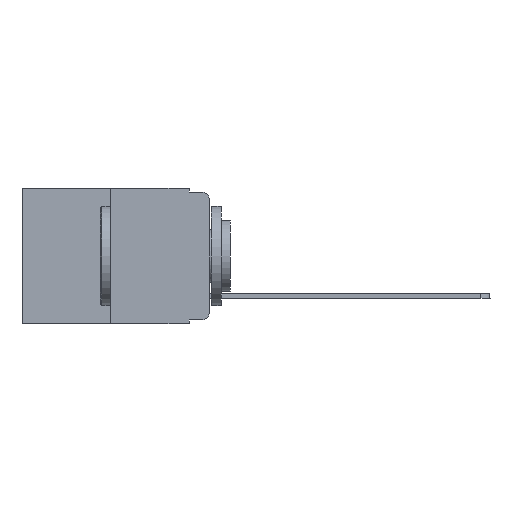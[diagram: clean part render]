
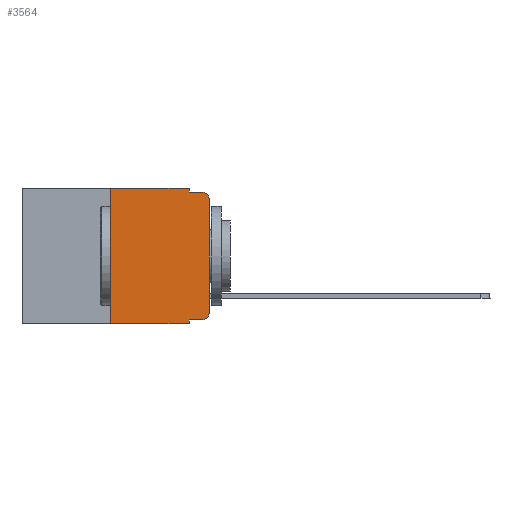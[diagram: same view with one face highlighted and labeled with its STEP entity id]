
A CAD part, left-side view. The second image highlights one B-rep face of the part: STEP entity #3564.
In plain terms, the highlighted planar face has unit normal (-1, 0, 0).
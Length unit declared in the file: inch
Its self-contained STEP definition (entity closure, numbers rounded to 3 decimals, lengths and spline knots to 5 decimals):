
#55 = ORIENTED_EDGE ( 'NONE', *, *, #7698, .F. ) ;
#363 = CARTESIAN_POINT ( 'NONE',  ( 0., 0.02, -0.313 ) ) ;
#516 = DIRECTION ( 'NONE',  ( 0., 0., -1. ) ) ;
#879 = VERTEX_POINT ( 'NONE', #20556 ) ;
#1262 = CIRCLE ( 'NONE', #7411, 0.02 ) ;
#1498 = CARTESIAN_POINT ( 'NONE',  ( 0., 0.051, -0.343 ) ) ;
#1668 = VECTOR ( 'NONE', #7666, 39.37008 ) ;
#1919 = DIRECTION ( 'NONE',  ( 0., 0., -1. ) ) ;
#2045 = CARTESIAN_POINT ( 'NONE',  ( 0., 0.473, 0. ) ) ;
#2085 = LINE ( 'NONE', #14810, #14218 ) ;
#2199 = ORIENTED_EDGE ( 'NONE', *, *, #12230, .T. ) ;
#2717 = EDGE_CURVE ( 'NONE', #3328, #7570, #13363, .T. ) ;
#3170 = CARTESIAN_POINT ( 'NONE',  ( 0., 0.051, 0. ) ) ;
#3328 = VERTEX_POINT ( 'NONE', #12734 ) ;
#3375 = VERTEX_POINT ( 'NONE', #3170 ) ;
#3502 = VECTOR ( 'NONE', #12272, 39.37008 ) ;
#3564 = ADVANCED_FACE ( 'NONE', ( #11796 ), #20050, .F. ) ;
#3728 = DIRECTION ( 'NONE',  ( 0., 0., -1. ) ) ;
#3743 = VECTOR ( 'NONE', #20815, 39.37008 ) ;
#4273 = VERTEX_POINT ( 'NONE', #11791 ) ;
#4708 = CARTESIAN_POINT ( 'NONE',  ( 0., 0., -0.313 ) ) ;
#4723 = EDGE_CURVE ( 'NONE', #5769, #3375, #13840, .T. ) ;
#4939 = CARTESIAN_POINT ( 'NONE',  ( 0., 0.02, -0.333 ) ) ;
#5488 = DIRECTION ( 'NONE',  ( 0., -1., 0. ) ) ;
#5769 = VERTEX_POINT ( 'NONE', #16128 ) ;
#6280 = VECTOR ( 'NONE', #12240, 39.37008 ) ;
#6304 = ORIENTED_EDGE ( 'NONE', *, *, #12163, .T. ) ;
#6412 = VERTEX_POINT ( 'NONE', #4939 ) ;
#6556 = LINE ( 'NONE', #14174, #15703 ) ;
#6940 = AXIS2_PLACEMENT_3D ( 'NONE', #2045, #8621, #516 ) ;
#7411 = AXIS2_PLACEMENT_3D ( 'NONE', #363, #11793, #3728 ) ;
#7445 = ORIENTED_EDGE ( 'NONE', *, *, #4723, .F. ) ;
#7570 = VERTEX_POINT ( 'NONE', #19523 ) ;
#7606 = LINE ( 'NONE', #7656, #7843 ) ;
#7656 = CARTESIAN_POINT ( 'NONE',  ( 0., 0.473, -0.343 ) ) ;
#7666 = DIRECTION ( 'NONE',  ( 0., -1., 0. ) ) ;
#7698 = EDGE_CURVE ( 'NONE', #3375, #3328, #2085, .T. ) ;
#7843 = VECTOR ( 'NONE', #19359, 39.37008 ) ;
#7973 = CARTESIAN_POINT ( 'NONE',  ( 0., 0.051, 0. ) ) ;
#8354 = DIRECTION ( 'NONE',  ( -1., 0., 0. ) ) ;
#8621 = DIRECTION ( 'NONE',  ( 1., 0., 0. ) ) ;
#8984 = EDGE_CURVE ( 'NONE', #6412, #18325, #1262, .T. ) ;
#9764 = DIRECTION ( 'NONE',  ( 0., 0., -1. ) ) ;
#10738 = ORIENTED_EDGE ( 'NONE', *, *, #17633, .F. ) ;
#11787 = ORIENTED_EDGE ( 'NONE', *, *, #2717, .F. ) ;
#11791 = CARTESIAN_POINT ( 'NONE',  ( 0., 0.051, -0.333 ) ) ;
#11793 = DIRECTION ( 'NONE',  ( -1., 0., 0. ) ) ;
#11796 = FACE_OUTER_BOUND ( 'NONE', #14832, .T. ) ;
#12132 = LINE ( 'NONE', #18901, #3502 ) ;
#12163 = EDGE_CURVE ( 'NONE', #4273, #6412, #6556, .T. ) ;
#12169 = CARTESIAN_POINT ( 'NONE',  ( 0., 0.051, -0.01 ) ) ;
#12230 = EDGE_CURVE ( 'NONE', #879, #12680, #7606, .T. ) ;
#12240 = DIRECTION ( 'NONE',  ( 0., 0., -1. ) ) ;
#12272 = DIRECTION ( 'NONE',  ( 0., 0., 1. ) ) ;
#12350 = LINE ( 'NONE', #17798, #3743 ) ;
#12552 = CARTESIAN_POINT ( 'NONE',  ( 0., 0.473, 0. ) ) ;
#12680 = VERTEX_POINT ( 'NONE', #1498 ) ;
#12729 = EDGE_CURVE ( 'NONE', #4273, #12680, #19195, .T. ) ;
#12734 = CARTESIAN_POINT ( 'NONE',  ( 0., 0.051, -0.01 ) ) ;
#13363 = LINE ( 'NONE', #12169, #19907 ) ;
#13840 = LINE ( 'NONE', #12552, #1668 ) ;
#14174 = CARTESIAN_POINT ( 'NONE',  ( 0., 0.051, -0.333 ) ) ;
#14218 = VECTOR ( 'NONE', #1919, 39.37008 ) ;
#14788 = ORIENTED_EDGE ( 'NONE', *, *, #18358, .T. ) ;
#14810 = CARTESIAN_POINT ( 'NONE',  ( 0., 0.051, 0. ) ) ;
#14832 = EDGE_LOOP ( 'NONE', ( #14788, #20108, #11787, #55, #7445, #10738, #2199, #20870, #6304, #17931 ) ) ;
#15673 = CARTESIAN_POINT ( 'NONE',  ( 0., 0., -0.03 ) ) ;
#15703 = VECTOR ( 'NONE', #20568, 39.37008 ) ;
#16128 = CARTESIAN_POINT ( 'NONE',  ( 0., 0.25, 0. ) ) ;
#17633 = EDGE_CURVE ( 'NONE', #879, #5769, #12132, .T. ) ;
#17680 = AXIS2_PLACEMENT_3D ( 'NONE', #18039, #8354, #9764 ) ;
#17798 = CARTESIAN_POINT ( 'NONE',  ( 0., 0., 0. ) ) ;
#17807 = EDGE_CURVE ( 'NONE', #18910, #7570, #20667, .T. ) ;
#17931 = ORIENTED_EDGE ( 'NONE', *, *, #8984, .T. ) ;
#18039 = CARTESIAN_POINT ( 'NONE',  ( 0., 0.02, -0.03 ) ) ;
#18325 = VERTEX_POINT ( 'NONE', #4708 ) ;
#18358 = EDGE_CURVE ( 'NONE', #18325, #18910, #12350, .T. ) ;
#18901 = CARTESIAN_POINT ( 'NONE',  ( 0., 0.25, 0. ) ) ;
#18910 = VERTEX_POINT ( 'NONE', #15673 ) ;
#19195 = LINE ( 'NONE', #7973, #6280 ) ;
#19359 = DIRECTION ( 'NONE',  ( 0., -1., 0. ) ) ;
#19523 = CARTESIAN_POINT ( 'NONE',  ( 0., 0.02, -0.01 ) ) ;
#19907 = VECTOR ( 'NONE', #5488, 39.37008 ) ;
#20050 = PLANE ( 'NONE',  #6940 ) ;
#20108 = ORIENTED_EDGE ( 'NONE', *, *, #17807, .T. ) ;
#20556 = CARTESIAN_POINT ( 'NONE',  ( 0., 0.25, -0.343 ) ) ;
#20568 = DIRECTION ( 'NONE',  ( 0., -1., 0. ) ) ;
#20667 = CIRCLE ( 'NONE', #17680, 0.02 ) ;
#20815 = DIRECTION ( 'NONE',  ( 0., 0., 1. ) ) ;
#20870 = ORIENTED_EDGE ( 'NONE', *, *, #12729, .F. ) ;
